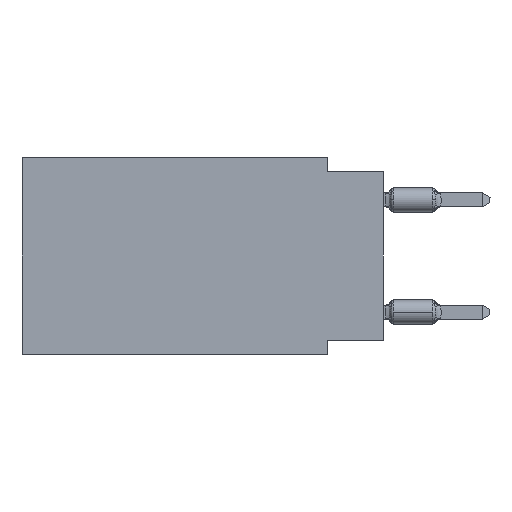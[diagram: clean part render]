
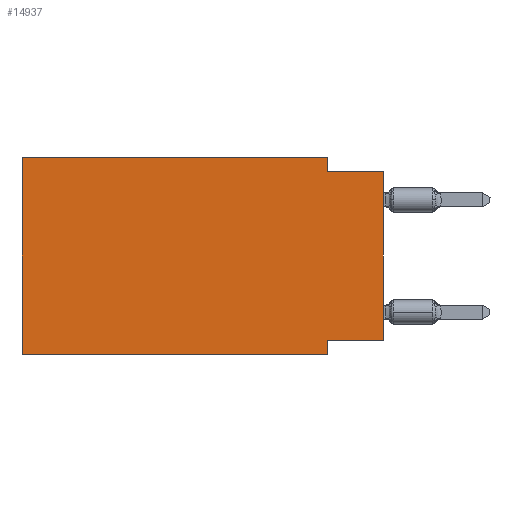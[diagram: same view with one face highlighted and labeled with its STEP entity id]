
A CAD part, left-side view. The second image highlights one B-rep face of the part: STEP entity #14937.
In plain terms, the highlighted planar face has unit normal (-1, 0, 0).
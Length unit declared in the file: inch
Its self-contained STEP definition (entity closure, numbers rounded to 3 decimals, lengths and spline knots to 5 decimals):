
#1227 = LINE ( 'NONE', #21405, #21478 ) ;
#2337 = DIRECTION ( 'NONE',  ( 1., 0., 0. ) ) ;
#2665 = ORIENTED_EDGE ( 'NONE', *, *, #16733, .F. ) ;
#2764 = VECTOR ( 'NONE', #30796, 39.37008 ) ;
#4240 = EDGE_CURVE ( 'NONE', #49410, #31753, #1227, .T. ) ;
#4498 = DIRECTION ( 'NONE',  ( 0., 0., -1. ) ) ;
#6647 = CARTESIAN_POINT ( 'NONE',  ( 0., 0.645, 0. ) ) ;
#6828 = CARTESIAN_POINT ( 'NONE',  ( 0., 0.1, -0.325 ) ) ;
#7753 = CARTESIAN_POINT ( 'NONE',  ( 0., 0.1, -0.35 ) ) ;
#8197 = EDGE_CURVE ( 'NONE', #27077, #49410, #24442, .T. ) ;
#10282 = DIRECTION ( 'NONE',  ( 0., -1., 0. ) ) ;
#11509 = VECTOR ( 'NONE', #4498, 39.37008 ) ;
#13953 = CARTESIAN_POINT ( 'NONE',  ( 0., 0.645, -0.35 ) ) ;
#14071 = CARTESIAN_POINT ( 'NONE',  ( 0., 0.645, 0. ) ) ;
#14937 = ADVANCED_FACE ( 'NONE', ( #29455 ), #37654, .F. ) ;
#15076 = CARTESIAN_POINT ( 'NONE',  ( 0., 0.645, -0.35 ) ) ;
#16733 = EDGE_CURVE ( 'NONE', #20091, #26229, #40237, .T. ) ;
#18379 = VECTOR ( 'NONE', #10282, 39.37008 ) ;
#20091 = VERTEX_POINT ( 'NONE', #29093 ) ;
#20411 = EDGE_LOOP ( 'NONE', ( #46424, #40963, #39259, #31066, #50006, #46652, #31669, #2665 ) ) ;
#21405 = CARTESIAN_POINT ( 'NONE',  ( 0., 0., -0.025 ) ) ;
#21478 = VECTOR ( 'NONE', #33636, 39.37008 ) ;
#22673 = EDGE_CURVE ( 'NONE', #45559, #27077, #29748, .T. ) ;
#22945 = VECTOR ( 'NONE', #26558, 39.37008 ) ;
#23540 = DIRECTION ( 'NONE',  ( 0., 1., 0. ) ) ;
#23713 = LINE ( 'NONE', #7753, #30576 ) ;
#24442 = LINE ( 'NONE', #49142, #11509 ) ;
#26229 = VERTEX_POINT ( 'NONE', #6828 ) ;
#26249 = EDGE_CURVE ( 'NONE', #32543, #41091, #47465, .T. ) ;
#26558 = DIRECTION ( 'NONE',  ( 0., 0., 1. ) ) ;
#27077 = VERTEX_POINT ( 'NONE', #32431 ) ;
#27451 = VECTOR ( 'NONE', #46718, 39.37008 ) ;
#28176 = AXIS2_PLACEMENT_3D ( 'NONE', #29711, #2337, #46686 ) ;
#28371 = EDGE_CURVE ( 'NONE', #26229, #41091, #23713, .T. ) ;
#28482 = DIRECTION ( 'NONE',  ( 0., 0., -1. ) ) ;
#28719 = EDGE_CURVE ( 'NONE', #32543, #45559, #42754, .T. ) ;
#29093 = CARTESIAN_POINT ( 'NONE',  ( 0., 0., -0.325 ) ) ;
#29455 = FACE_OUTER_BOUND ( 'NONE', #20411, .T. ) ;
#29711 = CARTESIAN_POINT ( 'NONE',  ( 0., 0.645, 0. ) ) ;
#29748 = LINE ( 'NONE', #14071, #27451 ) ;
#30175 = CARTESIAN_POINT ( 'NONE',  ( 0., 0.645, 0. ) ) ;
#30481 = EDGE_CURVE ( 'NONE', #20091, #31753, #49470, .T. ) ;
#30576 = VECTOR ( 'NONE', #28482, 39.37008 ) ;
#30796 = DIRECTION ( 'NONE',  ( 0., 0., 1. ) ) ;
#31066 = ORIENTED_EDGE ( 'NONE', *, *, #22673, .F. ) ;
#31669 = ORIENTED_EDGE ( 'NONE', *, *, #28371, .F. ) ;
#31753 = VERTEX_POINT ( 'NONE', #42287 ) ;
#32282 = CARTESIAN_POINT ( 'NONE',  ( 0., 0., -0.325 ) ) ;
#32431 = CARTESIAN_POINT ( 'NONE',  ( 0., 0.1, 0. ) ) ;
#32543 = VERTEX_POINT ( 'NONE', #13953 ) ;
#33636 = DIRECTION ( 'NONE',  ( 0., -1., 0. ) ) ;
#34527 = CARTESIAN_POINT ( 'NONE',  ( 0., 0., 0. ) ) ;
#35650 = CARTESIAN_POINT ( 'NONE',  ( 0., 0.1, -0.025 ) ) ;
#37654 = PLANE ( 'NONE',  #28176 ) ;
#38905 = CARTESIAN_POINT ( 'NONE',  ( 0., 0.1, -0.35 ) ) ;
#39259 = ORIENTED_EDGE ( 'NONE', *, *, #8197, .F. ) ;
#40215 = VECTOR ( 'NONE', #23540, 39.37008 ) ;
#40237 = LINE ( 'NONE', #32282, #40215 ) ;
#40963 = ORIENTED_EDGE ( 'NONE', *, *, #4240, .F. ) ;
#41091 = VERTEX_POINT ( 'NONE', #38905 ) ;
#42287 = CARTESIAN_POINT ( 'NONE',  ( 0., 0., -0.025 ) ) ;
#42754 = LINE ( 'NONE', #6647, #22945 ) ;
#45559 = VERTEX_POINT ( 'NONE', #30175 ) ;
#46424 = ORIENTED_EDGE ( 'NONE', *, *, #30481, .T. ) ;
#46652 = ORIENTED_EDGE ( 'NONE', *, *, #26249, .T. ) ;
#46686 = DIRECTION ( 'NONE',  ( 0., 0., -1. ) ) ;
#46718 = DIRECTION ( 'NONE',  ( 0., -1., 0. ) ) ;
#47465 = LINE ( 'NONE', #15076, #18379 ) ;
#49142 = CARTESIAN_POINT ( 'NONE',  ( 0., 0.1, 0. ) ) ;
#49410 = VERTEX_POINT ( 'NONE', #35650 ) ;
#49470 = LINE ( 'NONE', #34527, #2764 ) ;
#50006 = ORIENTED_EDGE ( 'NONE', *, *, #28719, .F. ) ;
